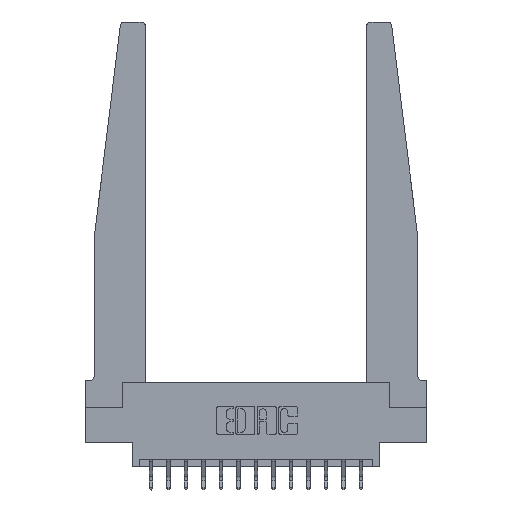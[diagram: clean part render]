
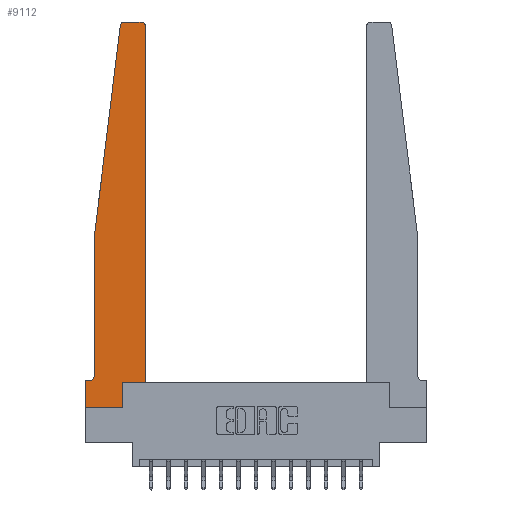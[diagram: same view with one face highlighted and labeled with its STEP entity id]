
A CAD part, top view. The second image highlights one B-rep face of the part: STEP entity #9112.
In plain terms, the highlighted planar face has unit normal (0, 0, 1).
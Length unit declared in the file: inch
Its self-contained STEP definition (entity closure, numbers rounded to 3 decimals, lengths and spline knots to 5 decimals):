
#8 = VECTOR ( 'NONE', #2452, 39.37008 ) ;
#90 = LINE ( 'NONE', #134, #3751 ) ;
#121 = LINE ( 'NONE', #1762, #4860 ) ;
#134 = CARTESIAN_POINT ( 'NONE',  ( 0., 0., 0.37 ) ) ;
#272 = ORIENTED_EDGE ( 'NONE', *, *, #5664, .T. ) ;
#641 = CARTESIAN_POINT ( 'NONE',  ( 0.2605, 0.18, 0.37 ) ) ;
#1168 = CARTESIAN_POINT ( 'NONE',  ( 0.065, 0.2375, 0.37 ) ) ;
#1394 = VECTOR ( 'NONE', #2149, 39.37008 ) ;
#1428 = AXIS2_PLACEMENT_3D ( 'NONE', #5446, #14892, #6797 ) ;
#1474 = VERTEX_POINT ( 'NONE', #5586 ) ;
#1667 = CIRCLE ( 'NONE', #14374, 0.03 ) ;
#1762 = CARTESIAN_POINT ( 'NONE',  ( 0., 0., 0.37 ) ) ;
#1817 = LINE ( 'NONE', #4917, #1394 ) ;
#1995 = ORIENTED_EDGE ( 'NONE', *, *, #2437, .T. ) ;
#2146 = AXIS2_PLACEMENT_3D ( 'NONE', #7097, #16497, #8450 ) ;
#2149 = DIRECTION ( 'NONE',  ( -0.122, -0.992, 0. ) ) ;
#2437 = EDGE_CURVE ( 'NONE', #2821, #16233, #5087, .T. ) ;
#2452 = DIRECTION ( 'NONE',  ( 1., 0., 0. ) ) ;
#2663 = EDGE_CURVE ( 'NONE', #3191, #5006, #121, .T. ) ;
#2821 = VERTEX_POINT ( 'NONE', #3488 ) ;
#3191 = VERTEX_POINT ( 'NONE', #8306 ) ;
#3269 = VECTOR ( 'NONE', #9793, 39.37008 ) ;
#3358 = DIRECTION ( 'NONE',  ( 0., 0., 1. ) ) ;
#3427 = ORIENTED_EDGE ( 'NONE', *, *, #6760, .T. ) ;
#3473 = CARTESIAN_POINT ( 'NONE',  ( 0.065, 0.1875, 0.37 ) ) ;
#3488 = CARTESIAN_POINT ( 'NONE',  ( 0.27653, 2.75, 0.37 ) ) ;
#3492 = VERTEX_POINT ( 'NONE', #16942 ) ;
#3504 = EDGE_CURVE ( 'NONE', #14392, #1474, #13706, .T. ) ;
#3579 = VERTEX_POINT ( 'NONE', #17108 ) ;
#3751 = VECTOR ( 'NONE', #13701, 39.37008 ) ;
#3876 = ORIENTED_EDGE ( 'NONE', *, *, #7578, .T. ) ;
#4117 = EDGE_CURVE ( 'NONE', #16233, #3579, #1817, .T. ) ;
#4134 = CARTESIAN_POINT ( 'NONE',  ( 0.2605, 0., 0.37 ) ) ;
#4280 = DIRECTION ( 'NONE',  ( -1., 0., 0. ) ) ;
#4408 = EDGE_CURVE ( 'NONE', #8337, #14392, #15177, .T. ) ;
#4860 = VECTOR ( 'NONE', #5912, 39.37008 ) ;
#4871 = EDGE_LOOP ( 'NONE', ( #272, #1995, #12393, #9679, #6087, #7580, #5871, #17367, #6900, #3427, #3876, #14523 ) ) ;
#4917 = CARTESIAN_POINT ( 'NONE',  ( 0.065, 1.25, 0.37 ) ) ;
#5006 = VERTEX_POINT ( 'NONE', #4134 ) ;
#5087 = CIRCLE ( 'NONE', #1428, 0.03 ) ;
#5434 = LINE ( 'NONE', #9693, #12616 ) ;
#5446 = CARTESIAN_POINT ( 'NONE',  ( 0.27653, 2.72, 0.37 ) ) ;
#5586 = CARTESIAN_POINT ( 'NONE',  ( 0., 0.1875, 0.37 ) ) ;
#5664 = EDGE_CURVE ( 'NONE', #3492, #2821, #5434, .T. ) ;
#5871 = ORIENTED_EDGE ( 'NONE', *, *, #16336, .T. ) ;
#5912 = DIRECTION ( 'NONE',  ( 1., 0., 0. ) ) ;
#6087 = ORIENTED_EDGE ( 'NONE', *, *, #4408, .T. ) ;
#6532 = CARTESIAN_POINT ( 'NONE',  ( 0.425, 0.18, 0.37 ) ) ;
#6542 = VECTOR ( 'NONE', #14339, 39.37008 ) ;
#6760 = EDGE_CURVE ( 'NONE', #12592, #14941, #14494, .T. ) ;
#6797 = DIRECTION ( 'NONE',  ( 1., 0., 0. ) ) ;
#6900 = ORIENTED_EDGE ( 'NONE', *, *, #12041, .T. ) ;
#7059 = LINE ( 'NONE', #11546, #13405 ) ;
#7097 = CARTESIAN_POINT ( 'NONE',  ( 0.015, 0.2375, 0.37 ) ) ;
#7578 = EDGE_CURVE ( 'NONE', #14941, #8202, #7059, .T. ) ;
#7580 = ORIENTED_EDGE ( 'NONE', *, *, #3504, .T. ) ;
#7732 = VECTOR ( 'NONE', #7773, 39.37008 ) ;
#7773 = DIRECTION ( 'NONE',  ( 0., -1., 0. ) ) ;
#8202 = VERTEX_POINT ( 'NONE', #10341 ) ;
#8306 = CARTESIAN_POINT ( 'NONE',  ( 0., 0., 0.37 ) ) ;
#8337 = VERTEX_POINT ( 'NONE', #1168 ) ;
#8450 = DIRECTION ( 'NONE',  ( -1., 0., 0. ) ) ;
#8706 = EDGE_CURVE ( 'NONE', #8202, #3492, #1667, .T. ) ;
#8916 = CARTESIAN_POINT ( 'NONE',  ( 0.015, 0.1875, 0.37 ) ) ;
#9112 = ADVANCED_FACE ( 'NONE', ( #9781 ), #14856, .T. ) ;
#9504 = DIRECTION ( 'NONE',  ( 1., 0., 0. ) ) ;
#9679 = ORIENTED_EDGE ( 'NONE', *, *, #13335, .T. ) ;
#9693 = CARTESIAN_POINT ( 'NONE',  ( 0.25, 2.75, 0.37 ) ) ;
#9781 = FACE_OUTER_BOUND ( 'NONE', #4871, .T. ) ;
#9793 = DIRECTION ( 'NONE',  ( 0., 1., 0. ) ) ;
#10341 = CARTESIAN_POINT ( 'NONE',  ( 0.425, 2.72, 0.37 ) ) ;
#10881 = LINE ( 'NONE', #15830, #7732 ) ;
#11421 = CARTESIAN_POINT ( 'NONE',  ( 0.425, 0.18, 0.37 ) ) ;
#11505 = CARTESIAN_POINT ( 'NONE',  ( 0.395, 2.72, 0.37 ) ) ;
#11546 = CARTESIAN_POINT ( 'NONE',  ( 0.425, 0.18, 0.37 ) ) ;
#12041 = EDGE_CURVE ( 'NONE', #5006, #12592, #13679, .T. ) ;
#12393 = ORIENTED_EDGE ( 'NONE', *, *, #4117, .T. ) ;
#12592 = VERTEX_POINT ( 'NONE', #641 ) ;
#12616 = VECTOR ( 'NONE', #4280, 39.37008 ) ;
#12862 = DIRECTION ( 'NONE',  ( 1., 0., 0. ) ) ;
#12897 = DIRECTION ( 'NONE',  ( 0., 1., 0. ) ) ;
#13117 = AXIS2_PLACEMENT_3D ( 'NONE', #16179, #17500, #9504 ) ;
#13335 = EDGE_CURVE ( 'NONE', #3579, #8337, #10881, .T. ) ;
#13405 = VECTOR ( 'NONE', #12897, 39.37008 ) ;
#13679 = LINE ( 'NONE', #13843, #3269 ) ;
#13701 = DIRECTION ( 'NONE',  ( 0., -1., 0. ) ) ;
#13706 = LINE ( 'NONE', #3473, #6542 ) ;
#13843 = CARTESIAN_POINT ( 'NONE',  ( 0.2605, 0.18, 0.37 ) ) ;
#14339 = DIRECTION ( 'NONE',  ( -1., 0., 0. ) ) ;
#14374 = AXIS2_PLACEMENT_3D ( 'NONE', #11505, #3358, #12862 ) ;
#14392 = VERTEX_POINT ( 'NONE', #8916 ) ;
#14494 = LINE ( 'NONE', #6532, #8 ) ;
#14523 = ORIENTED_EDGE ( 'NONE', *, *, #8706, .T. ) ;
#14856 = PLANE ( 'NONE',  #13117 ) ;
#14892 = DIRECTION ( 'NONE',  ( 0., 0., 1. ) ) ;
#14941 = VERTEX_POINT ( 'NONE', #11421 ) ;
#15177 = CIRCLE ( 'NONE', #2146, 0.05 ) ;
#15830 = CARTESIAN_POINT ( 'NONE',  ( 0.065, 1.25, 0.37 ) ) ;
#16046 = CARTESIAN_POINT ( 'NONE',  ( 0.24675, 2.72367, 0.37 ) ) ;
#16179 = CARTESIAN_POINT ( 'NONE',  ( 0., 0.1875, 0.37 ) ) ;
#16233 = VERTEX_POINT ( 'NONE', #16046 ) ;
#16336 = EDGE_CURVE ( 'NONE', #1474, #3191, #90, .T. ) ;
#16497 = DIRECTION ( 'NONE',  ( 0., 0., -1. ) ) ;
#16942 = CARTESIAN_POINT ( 'NONE',  ( 0.395, 2.75, 0.37 ) ) ;
#17108 = CARTESIAN_POINT ( 'NONE',  ( 0.065, 1.25, 0.37 ) ) ;
#17367 = ORIENTED_EDGE ( 'NONE', *, *, #2663, .T. ) ;
#17500 = DIRECTION ( 'NONE',  ( 0., 0., 1. ) ) ;
